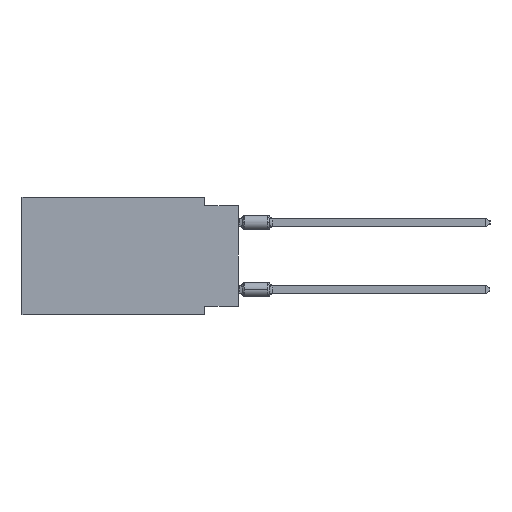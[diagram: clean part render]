
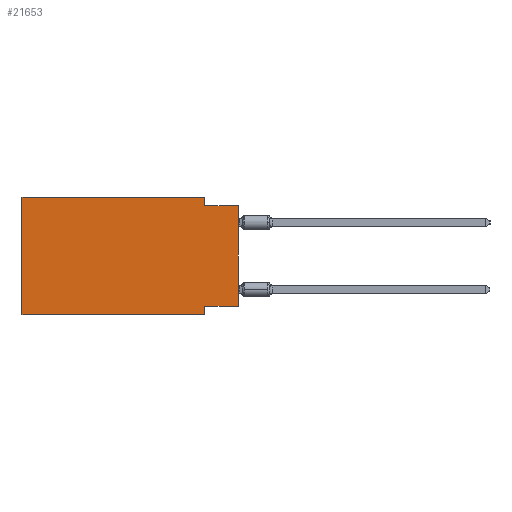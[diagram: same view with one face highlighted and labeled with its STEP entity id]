
A CAD part, left-side view. The second image highlights one B-rep face of the part: STEP entity #21653.
In plain terms, the highlighted planar face has unit normal (-1, 0, 0).
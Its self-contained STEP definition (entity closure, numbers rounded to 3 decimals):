
#505 = DIRECTION ( 'NONE',  ( 0., -1., 0. ) ) ;
#1257 = DIRECTION ( 'NONE',  ( 0., 0., 1. ) ) ;
#1287 = VERTEX_POINT ( 'NONE', #24403 ) ;
#2483 = EDGE_CURVE ( 'NONE', #4266, #32176, #28457, .T. ) ;
#2495 = PLANE ( 'NONE',  #31059 ) ;
#2906 = DIRECTION ( 'NONE',  ( 0., 0., -1. ) ) ;
#2914 = VERTEX_POINT ( 'NONE', #14220 ) ;
#3831 = DIRECTION ( 'NONE',  ( 0., 0., -1. ) ) ;
#4094 = VECTOR ( 'NONE', #5673, 1000. ) ;
#4266 = VERTEX_POINT ( 'NONE', #34366 ) ;
#4621 = VECTOR ( 'NONE', #3831, 1000. ) ;
#5590 = EDGE_CURVE ( 'NONE', #32176, #5759, #33131, .T. ) ;
#5673 = DIRECTION ( 'NONE',  ( 0., 0., 1. ) ) ;
#5759 = VERTEX_POINT ( 'NONE', #37203 ) ;
#10245 = LINE ( 'NONE', #34227, #25382 ) ;
#11126 = ORIENTED_EDGE ( 'NONE', *, *, #34015, .F. ) ;
#11194 = CARTESIAN_POINT ( 'NONE',  ( 0., 16.383, 0. ) ) ;
#11381 = DIRECTION ( 'NONE',  ( 1., 0., 0. ) ) ;
#11625 = ORIENTED_EDGE ( 'NONE', *, *, #21397, .F. ) ;
#11811 = LINE ( 'NONE', #35575, #4094 ) ;
#12258 = VERTEX_POINT ( 'NONE', #20494 ) ;
#12864 = VECTOR ( 'NONE', #1257, 1000. ) ;
#12894 = CARTESIAN_POINT ( 'NONE',  ( 0., 2.54, -8.89 ) ) ;
#13371 = VECTOR ( 'NONE', #21141, 1000. ) ;
#13491 = CARTESIAN_POINT ( 'NONE',  ( 0., 2.54, 0. ) ) ;
#13585 = VECTOR ( 'NONE', #25441, 1000. ) ;
#13727 = EDGE_CURVE ( 'NONE', #1287, #5759, #11811, .T. ) ;
#14220 = CARTESIAN_POINT ( 'NONE',  ( 0., 2.54, -8.89 ) ) ;
#14816 = ORIENTED_EDGE ( 'NONE', *, *, #32700, .F. ) ;
#14871 = EDGE_CURVE ( 'NONE', #12258, #2914, #34276, .T. ) ;
#16072 = LINE ( 'NONE', #34328, #29905 ) ;
#17001 = VECTOR ( 'NONE', #25500, 1000. ) ;
#19898 = ORIENTED_EDGE ( 'NONE', *, *, #2483, .F. ) ;
#20494 = CARTESIAN_POINT ( 'NONE',  ( 0., 16.383, -8.89 ) ) ;
#20690 = ORIENTED_EDGE ( 'NONE', *, *, #5590, .F. ) ;
#21141 = DIRECTION ( 'NONE',  ( 0., -1., 0. ) ) ;
#21397 = EDGE_CURVE ( 'NONE', #1287, #24262, #10245, .T. ) ;
#21532 = CARTESIAN_POINT ( 'NONE',  ( 0., 16.383, 0. ) ) ;
#21653 = ADVANCED_FACE ( 'NONE', ( #38277 ), #2495, .F. ) ;
#21922 = CARTESIAN_POINT ( 'NONE',  ( 0., 16.383, -8.89 ) ) ;
#22062 = DIRECTION ( 'NONE',  ( 0., 1., 0. ) ) ;
#24262 = VERTEX_POINT ( 'NONE', #34927 ) ;
#24403 = CARTESIAN_POINT ( 'NONE',  ( 0., 0., -8.255 ) ) ;
#25382 = VECTOR ( 'NONE', #22062, 1000. ) ;
#25441 = DIRECTION ( 'NONE',  ( 0., -1., 0. ) ) ;
#25500 = DIRECTION ( 'NONE',  ( 0., 0., -1. ) ) ;
#27468 = LINE ( 'NONE', #12894, #4621 ) ;
#28457 = LINE ( 'NONE', #13491, #17001 ) ;
#28762 = EDGE_CURVE ( 'NONE', #34946, #4266, #16072, .T. ) ;
#29905 = VECTOR ( 'NONE', #505, 1000. ) ;
#31059 = AXIS2_PLACEMENT_3D ( 'NONE', #11194, #11381, #2906 ) ;
#31597 = ORIENTED_EDGE ( 'NONE', *, *, #28762, .F. ) ;
#32176 = VERTEX_POINT ( 'NONE', #32612 ) ;
#32612 = CARTESIAN_POINT ( 'NONE',  ( 0., 2.54, -0.635 ) ) ;
#32700 = EDGE_CURVE ( 'NONE', #24262, #2914, #27468, .T. ) ;
#33131 = LINE ( 'NONE', #33709, #13371 ) ;
#33709 = CARTESIAN_POINT ( 'NONE',  ( 0., 0., -0.635 ) ) ;
#34015 = EDGE_CURVE ( 'NONE', #12258, #34946, #34889, .T. ) ;
#34227 = CARTESIAN_POINT ( 'NONE',  ( 0., 0., -8.255 ) ) ;
#34276 = LINE ( 'NONE', #21922, #13585 ) ;
#34328 = CARTESIAN_POINT ( 'NONE',  ( 0., 16.383, 0. ) ) ;
#34366 = CARTESIAN_POINT ( 'NONE',  ( 0., 2.54, 0. ) ) ;
#34494 = CARTESIAN_POINT ( 'NONE',  ( 0., 16.383, 0. ) ) ;
#34889 = LINE ( 'NONE', #34494, #12864 ) ;
#34927 = CARTESIAN_POINT ( 'NONE',  ( 0., 2.54, -8.255 ) ) ;
#34946 = VERTEX_POINT ( 'NONE', #21532 ) ;
#35320 = ORIENTED_EDGE ( 'NONE', *, *, #14871, .T. ) ;
#35575 = CARTESIAN_POINT ( 'NONE',  ( 0., 0., 0. ) ) ;
#36021 = EDGE_LOOP ( 'NONE', ( #37050, #20690, #19898, #31597, #11126, #35320, #14816, #11625 ) ) ;
#37050 = ORIENTED_EDGE ( 'NONE', *, *, #13727, .T. ) ;
#37203 = CARTESIAN_POINT ( 'NONE',  ( 0., 0., -0.635 ) ) ;
#38277 = FACE_OUTER_BOUND ( 'NONE', #36021, .T. ) ;
